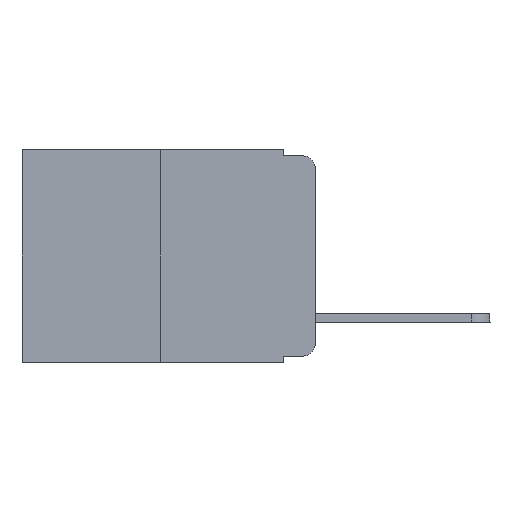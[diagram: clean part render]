
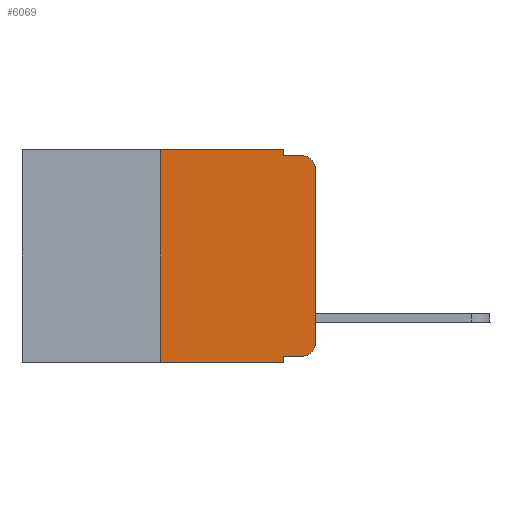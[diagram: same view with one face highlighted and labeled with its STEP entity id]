
A CAD part, left-side view. The second image highlights one B-rep face of the part: STEP entity #6069.
In plain terms, the highlighted planar face has unit normal (-1, 0, 0).
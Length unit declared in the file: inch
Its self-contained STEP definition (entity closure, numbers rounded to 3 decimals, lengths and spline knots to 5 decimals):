
#71 = DIRECTION ( 'NONE',  ( 0., 0., -1. ) ) ;
#101 = LINE ( 'NONE', #8432, #11045 ) ;
#372 = EDGE_CURVE ( 'NONE', #7054, #16997, #17006, .T. ) ;
#598 = CARTESIAN_POINT ( 'NONE',  ( 0., 0.25, -0.343 ) ) ;
#1291 = VECTOR ( 'NONE', #4370, 39.37008 ) ;
#1310 = CARTESIAN_POINT ( 'NONE',  ( 0., 0.473, 0. ) ) ;
#1733 = VECTOR ( 'NONE', #5457, 39.37008 ) ;
#2297 = LINE ( 'NONE', #14732, #10833 ) ;
#2430 = LINE ( 'NONE', #3911, #17486 ) ;
#2548 = FACE_OUTER_BOUND ( 'NONE', #15819, .T. ) ;
#3003 = VERTEX_POINT ( 'NONE', #598 ) ;
#3152 = CARTESIAN_POINT ( 'NONE',  ( 0., 0.051, -0.333 ) ) ;
#3681 = DIRECTION ( 'NONE',  ( -1., 0., 0. ) ) ;
#3911 = CARTESIAN_POINT ( 'NONE',  ( 0., 0.051, 0. ) ) ;
#3960 = CARTESIAN_POINT ( 'NONE',  ( 0., 0.02, -0.313 ) ) ;
#4370 = DIRECTION ( 'NONE',  ( 0., 0., 1. ) ) ;
#4481 = CARTESIAN_POINT ( 'NONE',  ( 0., 0., -0.03 ) ) ;
#4650 = ORIENTED_EDGE ( 'NONE', *, *, #12652, .T. ) ;
#5007 = VERTEX_POINT ( 'NONE', #10738 ) ;
#5457 = DIRECTION ( 'NONE',  ( 0., -1., 0. ) ) ;
#5719 = EDGE_CURVE ( 'NONE', #11612, #17657, #6985, .T. ) ;
#5749 = EDGE_CURVE ( 'NONE', #16997, #5007, #2430, .T. ) ;
#5885 = AXIS2_PLACEMENT_3D ( 'NONE', #6287, #3681, #16037 ) ;
#6069 = ADVANCED_FACE ( 'NONE', ( #2548 ), #12027, .F. ) ;
#6287 = CARTESIAN_POINT ( 'NONE',  ( 0., 0.02, -0.03 ) ) ;
#6410 = VERTEX_POINT ( 'NONE', #4481 ) ;
#6719 = ORIENTED_EDGE ( 'NONE', *, *, #5749, .F. ) ;
#6721 = LINE ( 'NONE', #9985, #17200 ) ;
#6820 = ORIENTED_EDGE ( 'NONE', *, *, #5719, .T. ) ;
#6887 = VECTOR ( 'NONE', #7847, 39.37008 ) ;
#6985 = CIRCLE ( 'NONE', #12703, 0.02 ) ;
#7054 = VERTEX_POINT ( 'NONE', #17246 ) ;
#7203 = VERTEX_POINT ( 'NONE', #3152 ) ;
#7289 = ORIENTED_EDGE ( 'NONE', *, *, #14722, .T. ) ;
#7522 = DIRECTION ( 'NONE',  ( 1., 0., 0. ) ) ;
#7719 = VERTEX_POINT ( 'NONE', #17369 ) ;
#7847 = DIRECTION ( 'NONE',  ( 0., -1., 0. ) ) ;
#8017 = AXIS2_PLACEMENT_3D ( 'NONE', #17949, #7522, #9020 ) ;
#8188 = EDGE_CURVE ( 'NONE', #7203, #7719, #101, .T. ) ;
#8281 = DIRECTION ( 'NONE',  ( -1., 0., 0. ) ) ;
#8432 = CARTESIAN_POINT ( 'NONE',  ( 0., 0.051, 0. ) ) ;
#8593 = ORIENTED_EDGE ( 'NONE', *, *, #372, .F. ) ;
#8865 = ORIENTED_EDGE ( 'NONE', *, *, #11456, .F. ) ;
#9020 = DIRECTION ( 'NONE',  ( 0., 0., -1. ) ) ;
#9304 = DIRECTION ( 'NONE',  ( 0., -1., 0. ) ) ;
#9417 = ORIENTED_EDGE ( 'NONE', *, *, #13174, .T. ) ;
#9697 = DIRECTION ( 'NONE',  ( 0., 0., -1. ) ) ;
#9985 = CARTESIAN_POINT ( 'NONE',  ( 0., 0.051, -0.333 ) ) ;
#10103 = CARTESIAN_POINT ( 'NONE',  ( 0., 0.25, 0. ) ) ;
#10587 = CARTESIAN_POINT ( 'NONE',  ( 0., 0.02, -0.333 ) ) ;
#10738 = CARTESIAN_POINT ( 'NONE',  ( 0., 0.051, -0.01 ) ) ;
#10833 = VECTOR ( 'NONE', #16116, 39.37008 ) ;
#10877 = DIRECTION ( 'NONE',  ( 0., 0., -1. ) ) ;
#11045 = VECTOR ( 'NONE', #71, 39.37008 ) ;
#11100 = VERTEX_POINT ( 'NONE', #13624 ) ;
#11456 = EDGE_CURVE ( 'NONE', #3003, #7054, #14183, .T. ) ;
#11612 = VERTEX_POINT ( 'NONE', #10587 ) ;
#11852 = VECTOR ( 'NONE', #9304, 39.37008 ) ;
#12027 = PLANE ( 'NONE',  #8017 ) ;
#12098 = CARTESIAN_POINT ( 'NONE',  ( 0., 0.051, 0. ) ) ;
#12478 = CIRCLE ( 'NONE', #5885, 0.02 ) ;
#12652 = EDGE_CURVE ( 'NONE', #3003, #7719, #15544, .T. ) ;
#12703 = AXIS2_PLACEMENT_3D ( 'NONE', #3960, #8281, #10877 ) ;
#12788 = DIRECTION ( 'NONE',  ( 0., -1., 0. ) ) ;
#13174 = EDGE_CURVE ( 'NONE', #6410, #11100, #12478, .T. ) ;
#13624 = CARTESIAN_POINT ( 'NONE',  ( 0., 0.02, -0.01 ) ) ;
#13674 = ORIENTED_EDGE ( 'NONE', *, *, #15863, .F. ) ;
#14183 = LINE ( 'NONE', #10103, #1291 ) ;
#14722 = EDGE_CURVE ( 'NONE', #7203, #11612, #6721, .T. ) ;
#14732 = CARTESIAN_POINT ( 'NONE',  ( 0., 0., 0. ) ) ;
#14755 = CARTESIAN_POINT ( 'NONE',  ( 0., 0.051, -0.01 ) ) ;
#14883 = CARTESIAN_POINT ( 'NONE',  ( 0., 0., -0.313 ) ) ;
#15544 = LINE ( 'NONE', #16316, #11852 ) ;
#15819 = EDGE_LOOP ( 'NONE', ( #17400, #9417, #13674, #6719, #8593, #8865, #4650, #16115, #7289, #6820 ) ) ;
#15863 = EDGE_CURVE ( 'NONE', #5007, #11100, #17153, .T. ) ;
#16037 = DIRECTION ( 'NONE',  ( 0., 0., -1. ) ) ;
#16115 = ORIENTED_EDGE ( 'NONE', *, *, #8188, .F. ) ;
#16116 = DIRECTION ( 'NONE',  ( 0., 0., 1. ) ) ;
#16316 = CARTESIAN_POINT ( 'NONE',  ( 0., 0.473, -0.343 ) ) ;
#16511 = EDGE_CURVE ( 'NONE', #17657, #6410, #2297, .T. ) ;
#16997 = VERTEX_POINT ( 'NONE', #12098 ) ;
#17006 = LINE ( 'NONE', #1310, #1733 ) ;
#17153 = LINE ( 'NONE', #14755, #6887 ) ;
#17200 = VECTOR ( 'NONE', #12788, 39.37008 ) ;
#17246 = CARTESIAN_POINT ( 'NONE',  ( 0., 0.25, 0. ) ) ;
#17369 = CARTESIAN_POINT ( 'NONE',  ( 0., 0.051, -0.343 ) ) ;
#17400 = ORIENTED_EDGE ( 'NONE', *, *, #16511, .T. ) ;
#17486 = VECTOR ( 'NONE', #9697, 39.37008 ) ;
#17657 = VERTEX_POINT ( 'NONE', #14883 ) ;
#17949 = CARTESIAN_POINT ( 'NONE',  ( 0., 0.473, 0. ) ) ;
